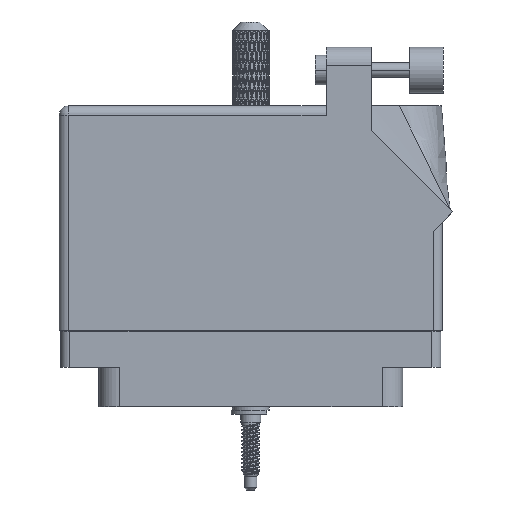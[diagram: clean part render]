
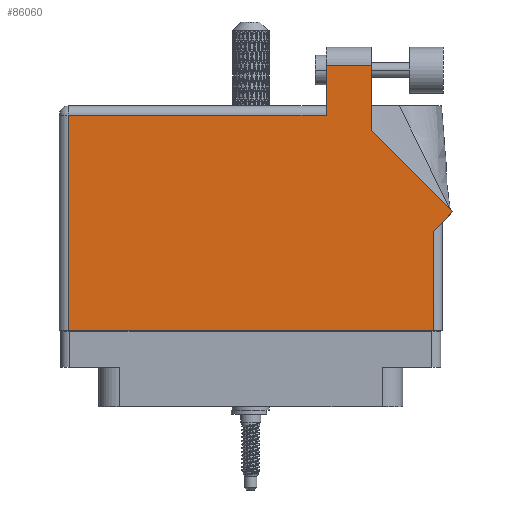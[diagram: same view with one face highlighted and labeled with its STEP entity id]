
A CAD part, front view. The second image highlights one B-rep face of the part: STEP entity #86060.
In plain terms, the highlighted face is planar.
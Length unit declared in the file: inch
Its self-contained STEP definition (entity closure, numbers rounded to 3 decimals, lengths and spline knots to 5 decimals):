
#2246 = LINE ( 'NONE', #39122, #100920 ) ;
#9268 = CARTESIAN_POINT ( 'NONE',  ( 0.513, 1.368, 0.455 ) ) ;
#9839 = CARTESIAN_POINT ( 'NONE',  ( 1.37671, 0.70771, 0.455 ) ) ;
#10518 = DIRECTION ( 'NONE',  ( 0., 1., 0. ) ) ;
#11120 = CARTESIAN_POINT ( 'NONE',  ( 1.244, 0.637, 0.455 ) ) ;
#11333 = CARTESIAN_POINT ( 'NONE',  ( 0.513, 1.705, 0.455 ) ) ;
#12654 = VECTOR ( 'NONE', #32238, 39.37008 ) ;
#12817 = VECTOR ( 'NONE', #10518, 39.37008 ) ;
#13167 = VECTOR ( 'NONE', #106937, 39.37008 ) ;
#15201 = VERTEX_POINT ( 'NONE', #52879 ) ;
#16080 = ORIENTED_EDGE ( 'NONE', *, *, #72872, .T. ) ;
#16642 = VECTOR ( 'NONE', #28261, 39.37008 ) ;
#17146 = VERTEX_POINT ( 'NONE', #51295 ) ;
#18767 = CARTESIAN_POINT ( 'NONE',  ( 1.37671, 0.70771, 0.455 ) ) ;
#20330 = CARTESIAN_POINT ( 'NONE',  ( -1.306, 1.43, 0.455 ) ) ;
#20630 = DIRECTION ( 'NONE',  ( 0.707, 0.707, 0. ) ) ;
#20847 = LINE ( 'NONE', #11333, #97252 ) ;
#21510 = DIRECTION ( 'NONE',  ( -1., 0., 0. ) ) ;
#25478 = AXIS2_PLACEMENT_3D ( 'NONE', #20330, #39950, #21510 ) ;
#27725 = CARTESIAN_POINT ( 'NONE',  ( 0.82, 1.26442, 0.455 ) ) ;
#28261 = DIRECTION ( 'NONE',  ( -0.707, 0.707, 0. ) ) ;
#30002 = ORIENTED_EDGE ( 'NONE', *, *, #39108, .T. ) ;
#30773 = EDGE_CURVE ( 'NONE', #70092, #111842, #101013, .T. ) ;
#31366 = DIRECTION ( 'NONE',  ( 1., 0., 0. ) ) ;
#32238 = DIRECTION ( 'NONE',  ( -1., 0., 0. ) ) ;
#32471 = EDGE_CURVE ( 'NONE', #64924, #82315, #85821, .T. ) ;
#34199 = CARTESIAN_POINT ( 'NONE',  ( 0.82, 1.705, 0.455 ) ) ;
#34573 = CARTESIAN_POINT ( 'NONE',  ( -1.244, -0.1, 0.455 ) ) ;
#38068 = EDGE_CURVE ( 'NONE', #15201, #64924, #59900, .T. ) ;
#39108 = EDGE_CURVE ( 'NONE', #17146, #79376, #72971, .T. ) ;
#39122 = CARTESIAN_POINT ( 'NONE',  ( -1.306, -0.1, 0.455 ) ) ;
#39950 = DIRECTION ( 'NONE',  ( 0., 0., -1. ) ) ;
#41379 = ORIENTED_EDGE ( 'NONE', *, *, #38068, .T. ) ;
#43503 = VERTEX_POINT ( 'NONE', #57698 ) ;
#44445 = CARTESIAN_POINT ( 'NONE',  ( 1.244, 0.575, 0.455 ) ) ;
#45071 = ORIENTED_EDGE ( 'NONE', *, *, #30773, .T. ) ;
#48008 = LINE ( 'NONE', #73604, #60719 ) ;
#51295 = CARTESIAN_POINT ( 'NONE',  ( 0.82, 1.26442, 0.455 ) ) ;
#52879 = CARTESIAN_POINT ( 'NONE',  ( 0.513, 1.705, 0.455 ) ) ;
#57139 = DIRECTION ( 'NONE',  ( -1., 0., 0. ) ) ;
#57698 = CARTESIAN_POINT ( 'NONE',  ( -1.244, -0.1, 0.455 ) ) ;
#59900 = LINE ( 'NONE', #113521, #13167 ) ;
#60719 = VECTOR ( 'NONE', #20630, 39.37008 ) ;
#63122 = LINE ( 'NONE', #34573, #69648 ) ;
#63362 = CARTESIAN_POINT ( 'NONE',  ( 1.244, -0.1, 0.455 ) ) ;
#63396 = LINE ( 'NONE', #9839, #16642 ) ;
#63509 = EDGE_LOOP ( 'NONE', ( #30002, #99677, #41379, #79156, #73381, #111703, #45071, #84669, #16080 ) ) ;
#64024 = DIRECTION ( 'NONE',  ( 0., 1., 0. ) ) ;
#64924 = VERTEX_POINT ( 'NONE', #9268 ) ;
#69374 = EDGE_CURVE ( 'NONE', #43503, #70092, #2246, .T. ) ;
#69648 = VECTOR ( 'NONE', #89341, 39.37008 ) ;
#70092 = VERTEX_POINT ( 'NONE', #63362 ) ;
#72872 = EDGE_CURVE ( 'NONE', #100075, #17146, #63396, .T. ) ;
#72971 = LINE ( 'NONE', #27725, #96500 ) ;
#73381 = ORIENTED_EDGE ( 'NONE', *, *, #73553, .T. ) ;
#73553 = EDGE_CURVE ( 'NONE', #82315, #43503, #63122, .T. ) ;
#73604 = CARTESIAN_POINT ( 'NONE',  ( 1.306, 0.637, 0.455 ) ) ;
#77534 = EDGE_CURVE ( 'NONE', #79376, #15201, #20847, .T. ) ;
#79156 = ORIENTED_EDGE ( 'NONE', *, *, #32471, .T. ) ;
#79376 = VERTEX_POINT ( 'NONE', #34199 ) ;
#82315 = VERTEX_POINT ( 'NONE', #109129 ) ;
#84669 = ORIENTED_EDGE ( 'NONE', *, *, #102357, .T. ) ;
#85821 = LINE ( 'NONE', #96516, #12654 ) ;
#86060 = ADVANCED_FACE ( 'NONE', ( #101867 ), #103064, .F. ) ;
#89341 = DIRECTION ( 'NONE',  ( 0., -1., 0. ) ) ;
#96500 = VECTOR ( 'NONE', #64024, 39.37008 ) ;
#96516 = CARTESIAN_POINT ( 'NONE',  ( -1.306, 1.368, 0.455 ) ) ;
#97252 = VECTOR ( 'NONE', #57139, 39.37008 ) ;
#99677 = ORIENTED_EDGE ( 'NONE', *, *, #77534, .T. ) ;
#100075 = VERTEX_POINT ( 'NONE', #18767 ) ;
#100920 = VECTOR ( 'NONE', #31366, 39.37008 ) ;
#101013 = LINE ( 'NONE', #11120, #12817 ) ;
#101867 = FACE_OUTER_BOUND ( 'NONE', #63509, .T. ) ;
#102357 = EDGE_CURVE ( 'NONE', #111842, #100075, #48008, .T. ) ;
#103064 = PLANE ( 'NONE',  #25478 ) ;
#106937 = DIRECTION ( 'NONE',  ( 0., -1., 0. ) ) ;
#109129 = CARTESIAN_POINT ( 'NONE',  ( -1.244, 1.368, 0.455 ) ) ;
#111703 = ORIENTED_EDGE ( 'NONE', *, *, #69374, .T. ) ;
#111842 = VERTEX_POINT ( 'NONE', #44445 ) ;
#113521 = CARTESIAN_POINT ( 'NONE',  ( 0.513, 1.43, 0.455 ) ) ;
